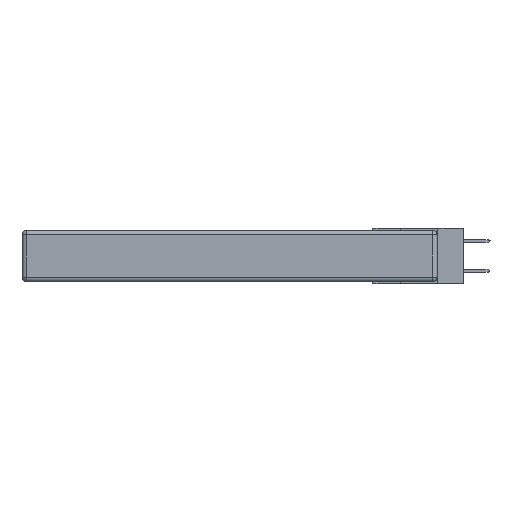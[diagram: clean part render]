
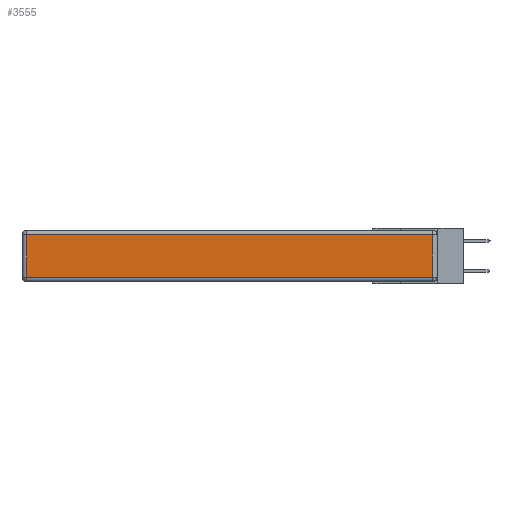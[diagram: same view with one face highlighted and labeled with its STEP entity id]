
A CAD part, left-side view. The second image highlights one B-rep face of the part: STEP entity #3555.
In plain terms, the highlighted planar face has unit normal (-1, 0, 0).
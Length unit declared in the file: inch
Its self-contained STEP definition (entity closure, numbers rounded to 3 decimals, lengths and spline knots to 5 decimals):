
#506 = CARTESIAN_POINT ( 'NONE',  ( 0., 0., -0.313 ) ) ;
#713 = VECTOR ( 'NONE', #17979, 39.37008 ) ;
#2198 = CARTESIAN_POINT ( 'NONE',  ( 0., 2.72, -0.03 ) ) ;
#2636 = DIRECTION ( 'NONE',  ( 0., 0., 1. ) ) ;
#3276 = DIRECTION ( 'NONE',  ( 0., 0., 1. ) ) ;
#3430 = EDGE_LOOP ( 'NONE', ( #17549, #9769, #5661, #24827 ) ) ;
#3555 = ADVANCED_FACE ( 'NONE', ( #13366 ), #24309, .T. ) ;
#3891 = LINE ( 'NONE', #506, #713 ) ;
#4897 = AXIS2_PLACEMENT_3D ( 'NONE', #30060, #17547, #2636 ) ;
#5656 = CARTESIAN_POINT ( 'NONE',  ( 0., 2.75, -0.03 ) ) ;
#5661 = ORIENTED_EDGE ( 'NONE', *, *, #16283, .T. ) ;
#5858 = CARTESIAN_POINT ( 'NONE',  ( 0., 2.72, -0.343 ) ) ;
#7447 = VECTOR ( 'NONE', #3276, 39.37008 ) ;
#8396 = EDGE_CURVE ( 'NONE', #26896, #23795, #31574, .T. ) ;
#8609 = DIRECTION ( 'NONE',  ( 0., 1., 0. ) ) ;
#9769 = ORIENTED_EDGE ( 'NONE', *, *, #23709, .T. ) ;
#10684 = CARTESIAN_POINT ( 'NONE',  ( 0., 0.03, -0.343 ) ) ;
#13217 = CARTESIAN_POINT ( 'NONE',  ( 0., 0.03, -0.03 ) ) ;
#13366 = FACE_OUTER_BOUND ( 'NONE', #3430, .T. ) ;
#13534 = DIRECTION ( 'NONE',  ( 0., 0., -1. ) ) ;
#14852 = CARTESIAN_POINT ( 'NONE',  ( 0., 0.03, -0.313 ) ) ;
#14957 = VERTEX_POINT ( 'NONE', #13217 ) ;
#16283 = EDGE_CURVE ( 'NONE', #14957, #26896, #24580, .T. ) ;
#16889 = EDGE_CURVE ( 'NONE', #23795, #21738, #3891, .T. ) ;
#17547 = DIRECTION ( 'NONE',  ( -1., 0., 0. ) ) ;
#17549 = ORIENTED_EDGE ( 'NONE', *, *, #16889, .T. ) ;
#17913 = VECTOR ( 'NONE', #13534, 39.37008 ) ;
#17979 = DIRECTION ( 'NONE',  ( 0., -1., 0. ) ) ;
#21738 = VERTEX_POINT ( 'NONE', #14852 ) ;
#21983 = CARTESIAN_POINT ( 'NONE',  ( 0., 2.72, -0.313 ) ) ;
#23041 = LINE ( 'NONE', #10684, #7447 ) ;
#23709 = EDGE_CURVE ( 'NONE', #21738, #14957, #23041, .T. ) ;
#23795 = VERTEX_POINT ( 'NONE', #21983 ) ;
#24309 = PLANE ( 'NONE',  #4897 ) ;
#24580 = LINE ( 'NONE', #5656, #30403 ) ;
#24827 = ORIENTED_EDGE ( 'NONE', *, *, #8396, .T. ) ;
#26896 = VERTEX_POINT ( 'NONE', #2198 ) ;
#30060 = CARTESIAN_POINT ( 'NONE',  ( 0., 0., -0.343 ) ) ;
#30403 = VECTOR ( 'NONE', #8609, 39.37008 ) ;
#31574 = LINE ( 'NONE', #5858, #17913 ) ;
